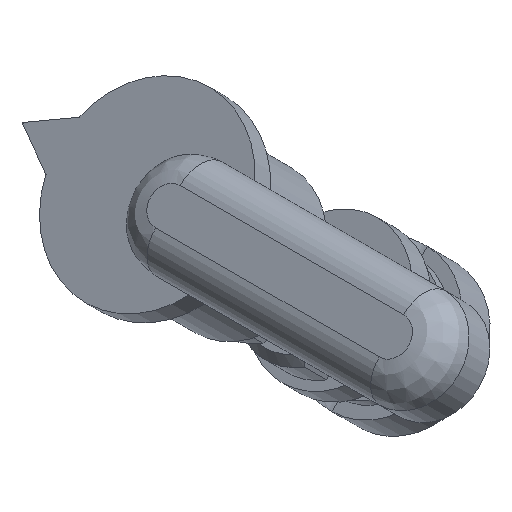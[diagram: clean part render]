
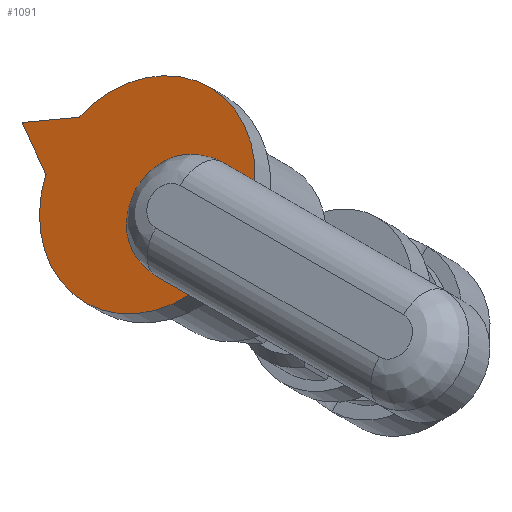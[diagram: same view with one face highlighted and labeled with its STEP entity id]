
A CAD part, isometric view. The second image highlights one B-rep face of the part: STEP entity #1091.
In plain terms, the highlighted planar face has unit normal (-0.707, 0, 0.707).
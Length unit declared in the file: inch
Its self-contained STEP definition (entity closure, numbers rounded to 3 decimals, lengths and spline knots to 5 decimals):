
#120=CIRCLE('',#1176,0.125);
#132=CIRCLE('',#1204,0.23622);
#134=CIRCLE('',#1207,0.23622);
#196=FACE_OUTER_BOUND('',#259,.T.);
#259=EDGE_LOOP('',(#921,#922,#923,#924,#925,#926,#927));
#324=LINE('',#1750,#400);
#338=LINE('',#2309,#414);
#341=LINE('',#2315,#417);
#344=LINE('',#2327,#420);
#400=VECTOR('',#1376,0.3937);
#414=VECTOR('',#1442,0.3937);
#417=VECTOR('',#1447,0.3937);
#420=VECTOR('',#1464,0.3937);
#490=VERTEX_POINT('',#1747);
#491=VERTEX_POINT('',#1749);
#494=VERTEX_POINT('',#1757);
#523=VERTEX_POINT('',#2306);
#524=VERTEX_POINT('',#2308);
#526=VERTEX_POINT('',#2314);
#528=VERTEX_POINT('',#2320);
#615=EDGE_CURVE('',#490,#491,#324,.T.);
#620=EDGE_CURVE('',#494,#490,#120,.T.);
#664=EDGE_CURVE('',#524,#523,#338,.T.);
#667=EDGE_CURVE('',#526,#524,#341,.T.);
#670=EDGE_CURVE('',#528,#526,#132,.T.);
#673=EDGE_CURVE('',#523,#491,#134,.T.);
#674=EDGE_CURVE('',#528,#494,#344,.T.);
#921=ORIENTED_EDGE('',*,*,#673,.T.);
#922=ORIENTED_EDGE('',*,*,#615,.F.);
#923=ORIENTED_EDGE('',*,*,#620,.F.);
#924=ORIENTED_EDGE('',*,*,#674,.F.);
#925=ORIENTED_EDGE('',*,*,#670,.T.);
#926=ORIENTED_EDGE('',*,*,#667,.T.);
#927=ORIENTED_EDGE('',*,*,#664,.T.);
#1035=PLANE('',#1208);
#1091=ADVANCED_FACE('',(#196),#1035,.T.);
#1176=AXIS2_PLACEMENT_3D('',#1759,#1383,#1384);
#1204=AXIS2_PLACEMENT_3D('',#2321,#1453,#1454);
#1207=AXIS2_PLACEMENT_3D('',#2325,#1460,#1461);
#1208=AXIS2_PLACEMENT_3D('',#2326,#1462,#1463);
#1376=DIRECTION('',(0.,-1.,0.));
#1383=DIRECTION('center_axis',(-0.707,0.,0.707));
#1384=DIRECTION('ref_axis',(0.707,0.,0.707));
#1442=DIRECTION('',(-0.354,-0.866,-0.354));
#1447=DIRECTION('',(-0.354,0.866,-0.354));
#1453=DIRECTION('center_axis',(-0.707,0.,0.707));
#1454=DIRECTION('ref_axis',(0.707,0.,0.707));
#1460=DIRECTION('center_axis',(-0.707,0.,0.707));
#1461=DIRECTION('ref_axis',(0.,-1.,0.));
#1462=DIRECTION('center_axis',(-0.707,0.,0.707));
#1463=DIRECTION('ref_axis',(0.707,0.,0.707));
#1464=DIRECTION('',(0.,1.,0.));
#1747=CARTESIAN_POINT('',(-0.11878,-0.125,0.07586));
#1749=CARTESIAN_POINT('',(-0.11878,-0.20044,0.07586));
#1750=CARTESIAN_POINT('',(-0.11878,-0.02855,0.07586));
#1757=CARTESIAN_POINT('',(0.058,-0.125,0.25264));
#1759=CARTESIAN_POINT('Origin',(-0.03039,-0.125,0.16425));
#2306=CARTESIAN_POINT('',(-0.07467,0.22777,0.11997));
#2308=CARTESIAN_POINT('',(-0.03039,0.33622,0.16425));
#2309=CARTESIAN_POINT('',(-0.03039,0.33622,0.16425));
#2314=CARTESIAN_POINT('',(0.01388,0.22777,0.20852));
#2315=CARTESIAN_POINT('',(0.01388,0.22777,0.20852));
#2320=CARTESIAN_POINT('',(0.058,-0.20044,0.25264));
#2321=CARTESIAN_POINT('Origin',(-0.03039,0.,0.16425));
#2325=CARTESIAN_POINT('Origin',(-0.03039,0.,0.16425));
#2326=CARTESIAN_POINT('Origin',(-0.0784,0.,0.11624));
#2327=CARTESIAN_POINT('',(0.058,-0.32855,0.25264));
